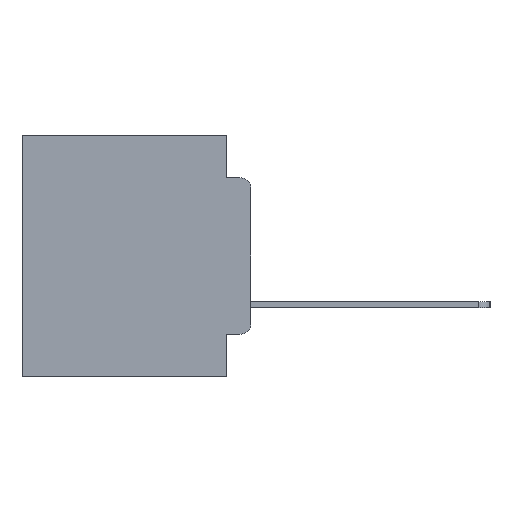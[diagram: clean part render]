
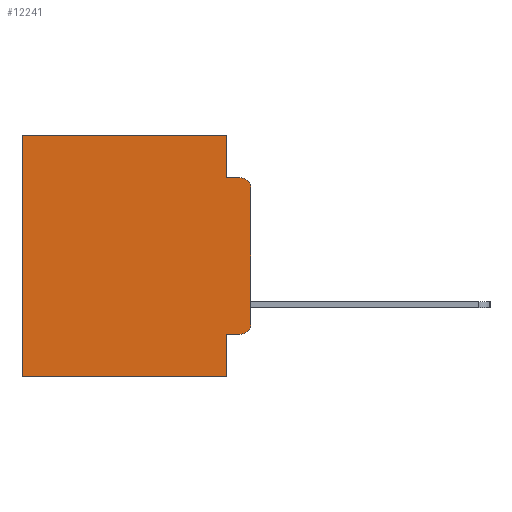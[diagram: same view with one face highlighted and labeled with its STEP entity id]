
A CAD part, left-side view. The second image highlights one B-rep face of the part: STEP entity #12241.
In plain terms, the highlighted planar face has unit normal (-1, 0, 0).
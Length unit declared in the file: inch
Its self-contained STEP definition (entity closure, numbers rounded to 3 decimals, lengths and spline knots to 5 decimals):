
#130 = LINE ( 'NONE', #14120, #11179 ) ;
#192 = VERTEX_POINT ( 'NONE', #10030 ) ;
#438 = ORIENTED_EDGE ( 'NONE', *, *, #15940, .F. ) ;
#1555 = ORIENTED_EDGE ( 'NONE', *, *, #17376, .F. ) ;
#2457 = DIRECTION ( 'NONE',  ( 0., 1., 0. ) ) ;
#2542 = AXIS2_PLACEMENT_3D ( 'NONE', #18631, #5807, #20738 ) ;
#3020 = LINE ( 'NONE', #18613, #24916 ) ;
#3220 = LINE ( 'NONE', #22587, #19069 ) ;
#4125 = VECTOR ( 'NONE', #9424, 39.37008 ) ;
#4856 = LINE ( 'NONE', #20134, #4125 ) ;
#5049 = LINE ( 'NONE', #21425, #26660 ) ;
#5807 = DIRECTION ( 'NONE',  ( 1., 0., 0. ) ) ;
#5852 = EDGE_CURVE ( 'NONE', #13119, #192, #11698, .T. ) ;
#6021 = AXIS2_PLACEMENT_3D ( 'NONE', #17035, #26827, #26858 ) ;
#6262 = VERTEX_POINT ( 'NONE', #7997 ) ;
#6601 = DIRECTION ( 'NONE',  ( 0., 0., -1. ) ) ;
#7452 = FACE_OUTER_BOUND ( 'NONE', #10861, .T. ) ;
#7899 = CARTESIAN_POINT ( 'NONE',  ( 0.298, 0.473, 0. ) ) ;
#7997 = CARTESIAN_POINT ( 'NONE',  ( 0.298, 0.051, 0. ) ) ;
#8039 = VERTEX_POINT ( 'NONE', #25606 ) ;
#8163 = ORIENTED_EDGE ( 'NONE', *, *, #5852, .T. ) ;
#8530 = LINE ( 'NONE', #11932, #13637 ) ;
#8646 = EDGE_CURVE ( 'NONE', #12773, #13119, #130, .T. ) ;
#8821 = CIRCLE ( 'NONE', #11421, 0.02 ) ;
#9129 = ORIENTED_EDGE ( 'NONE', *, *, #10032, .F. ) ;
#9424 = DIRECTION ( 'NONE',  ( 0., 0., -1. ) ) ;
#9898 = DIRECTION ( 'NONE',  ( 0., 0., -1. ) ) ;
#10030 = CARTESIAN_POINT ( 'NONE',  ( 0.298, 0., -0.3915 ) ) ;
#10032 = EDGE_CURVE ( 'NONE', #12773, #27576, #3020, .T. ) ;
#10440 = ORIENTED_EDGE ( 'NONE', *, *, #18764, .T. ) ;
#10486 = CARTESIAN_POINT ( 'NONE',  ( 0.298, 0.02, -0.1085 ) ) ;
#10861 = EDGE_LOOP ( 'NONE', ( #27113, #10440, #1555, #438, #11759, #25371, #11967, #9129, #20917, #8163 ) ) ;
#10925 = CARTESIAN_POINT ( 'NONE',  ( 0.298, 0., -0.1085 ) ) ;
#11179 = VECTOR ( 'NONE', #13782, 39.37008 ) ;
#11287 = VERTEX_POINT ( 'NONE', #17064 ) ;
#11421 = AXIS2_PLACEMENT_3D ( 'NONE', #10486, #25208, #12732 ) ;
#11521 = EDGE_CURVE ( 'NONE', #17453, #11995, #4856, .T. ) ;
#11698 = CIRCLE ( 'NONE', #6021, 0.02 ) ;
#11759 = ORIENTED_EDGE ( 'NONE', *, *, #22569, .T. ) ;
#11932 = CARTESIAN_POINT ( 'NONE',  ( 0.298, 0.051, -0.0885 ) ) ;
#11967 = ORIENTED_EDGE ( 'NONE', *, *, #13391, .F. ) ;
#11995 = VERTEX_POINT ( 'NONE', #13396 ) ;
#12241 = ADVANCED_FACE ( 'NONE', ( #7452 ), #24674, .F. ) ;
#12293 = CARTESIAN_POINT ( 'NONE',  ( 0.298, 0.051, -0.4115 ) ) ;
#12522 = VECTOR ( 'NONE', #2457, 39.37008 ) ;
#12732 = DIRECTION ( 'NONE',  ( 0., 0., -1. ) ) ;
#12773 = VERTEX_POINT ( 'NONE', #12293 ) ;
#13119 = VERTEX_POINT ( 'NONE', #19938 ) ;
#13196 = LINE ( 'NONE', #15486, #12522 ) ;
#13391 = EDGE_CURVE ( 'NONE', #27576, #11995, #13196, .T. ) ;
#13396 = CARTESIAN_POINT ( 'NONE',  ( 0.298, 0.473, -0.5 ) ) ;
#13637 = VECTOR ( 'NONE', #14180, 39.37008 ) ;
#13782 = DIRECTION ( 'NONE',  ( 0., -1., 0. ) ) ;
#14120 = CARTESIAN_POINT ( 'NONE',  ( 0.298, 0.051, -0.4115 ) ) ;
#14180 = DIRECTION ( 'NONE',  ( 0., -1., 0. ) ) ;
#15486 = CARTESIAN_POINT ( 'NONE',  ( 0.298, 0., -0.5 ) ) ;
#15940 = EDGE_CURVE ( 'NONE', #6262, #11287, #17109, .T. ) ;
#17035 = CARTESIAN_POINT ( 'NONE',  ( 0.298, 0.02, -0.3915 ) ) ;
#17064 = CARTESIAN_POINT ( 'NONE',  ( 0.298, 0.051, -0.0885 ) ) ;
#17109 = LINE ( 'NONE', #21509, #17780 ) ;
#17376 = EDGE_CURVE ( 'NONE', #11287, #8039, #8530, .T. ) ;
#17453 = VERTEX_POINT ( 'NONE', #7899 ) ;
#17780 = VECTOR ( 'NONE', #6601, 39.37008 ) ;
#18480 = DIRECTION ( 'NONE',  ( 0., 0., -1. ) ) ;
#18613 = CARTESIAN_POINT ( 'NONE',  ( 0.298, 0.051, 0. ) ) ;
#18631 = CARTESIAN_POINT ( 'NONE',  ( 0.298, 0., 0. ) ) ;
#18764 = EDGE_CURVE ( 'NONE', #19544, #8039, #8821, .T. ) ;
#19069 = VECTOR ( 'NONE', #18480, 39.37008 ) ;
#19544 = VERTEX_POINT ( 'NONE', #10925 ) ;
#19938 = CARTESIAN_POINT ( 'NONE',  ( 0.298, 0.02, -0.4115 ) ) ;
#20134 = CARTESIAN_POINT ( 'NONE',  ( 0.298, 0.473, 0. ) ) ;
#20738 = DIRECTION ( 'NONE',  ( 0., 0., -1. ) ) ;
#20917 = ORIENTED_EDGE ( 'NONE', *, *, #8646, .T. ) ;
#21331 = CARTESIAN_POINT ( 'NONE',  ( 0.298, 0.051, -0.5 ) ) ;
#21425 = CARTESIAN_POINT ( 'NONE',  ( 0.298, 0., 0. ) ) ;
#21509 = CARTESIAN_POINT ( 'NONE',  ( 0.298, 0.051, 0. ) ) ;
#22569 = EDGE_CURVE ( 'NONE', #6262, #17453, #5049, .T. ) ;
#22587 = CARTESIAN_POINT ( 'NONE',  ( 0.298, 0., 0. ) ) ;
#23516 = DIRECTION ( 'NONE',  ( 0., 1., 0. ) ) ;
#24224 = EDGE_CURVE ( 'NONE', #19544, #192, #3220, .T. ) ;
#24674 = PLANE ( 'NONE',  #2542 ) ;
#24916 = VECTOR ( 'NONE', #9898, 39.37008 ) ;
#25208 = DIRECTION ( 'NONE',  ( -1., 0., 0. ) ) ;
#25371 = ORIENTED_EDGE ( 'NONE', *, *, #11521, .T. ) ;
#25606 = CARTESIAN_POINT ( 'NONE',  ( 0.298, 0.02, -0.0885 ) ) ;
#26660 = VECTOR ( 'NONE', #23516, 39.37008 ) ;
#26827 = DIRECTION ( 'NONE',  ( -1., 0., 0. ) ) ;
#26858 = DIRECTION ( 'NONE',  ( 0., 0., -1. ) ) ;
#27113 = ORIENTED_EDGE ( 'NONE', *, *, #24224, .F. ) ;
#27576 = VERTEX_POINT ( 'NONE', #21331 ) ;
